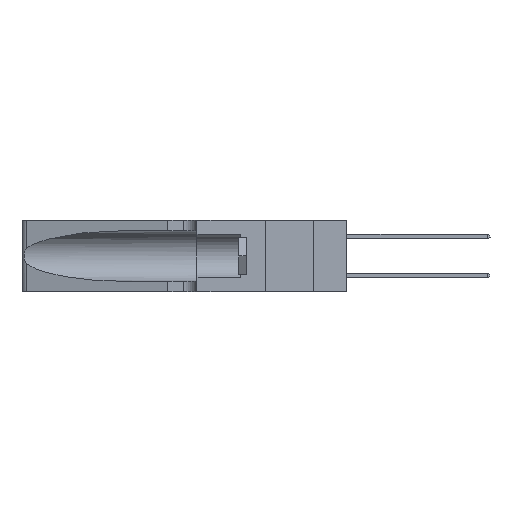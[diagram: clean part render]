
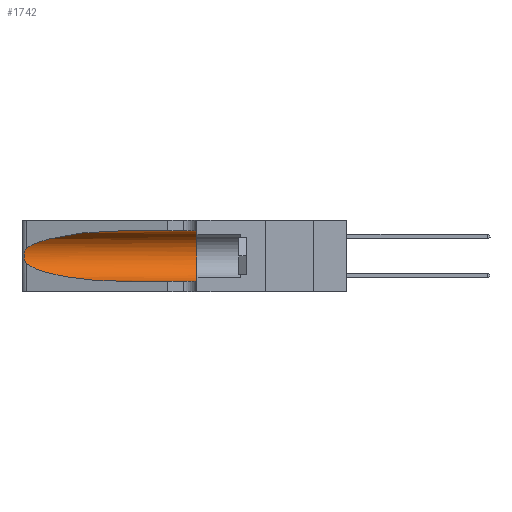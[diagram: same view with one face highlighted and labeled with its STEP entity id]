
A CAD part, left-side view. The second image highlights one B-rep face of the part: STEP entity #1742.
In plain terms, the highlighted cylindrical face has radius 3.308 mm (diameter 6.617 mm), a partial arc.
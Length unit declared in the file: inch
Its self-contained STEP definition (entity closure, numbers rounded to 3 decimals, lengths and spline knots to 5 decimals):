
#108 = CARTESIAN_POINT ( 'NONE',  ( 0.25487, 1.22718, 0.22369 ) ) ;
#180 = EDGE_CURVE ( 'NONE', #36147, #35010, #6862, .T. ) ;
#284 = DIRECTION ( 'NONE',  ( 0., -1., 0. ) ) ;
#450 = CARTESIAN_POINT ( 'NONE',  ( 0.25555, 1.22993, 0.14849 ) ) ;
#889 = B_SPLINE_CURVE_WITH_KNOTS ( 'NONE', 3,
 ( #3472, #22132, #25233, #6663, #28378, #9851, #31493, #12985, #34604, #16064, #37727, #19160, #450, #22259 ),
 .UNSPECIFIED., .F., .F.,
 ( 4, 2, 2, 2, 2, 2, 4 ),
 ( 0., 0.00027, 0.00053, 0.00107, 0.0016, 0.00187, 0.00214 ),
 .UNSPECIFIED. ) ;
#1436 = AXIS2_PLACEMENT_3D ( 'NONE', #6630, #284, #28343 ) ;
#1742 = ADVANCED_FACE ( 'NONE', ( #29060 ), #4242, .F. ) ;
#3472 = CARTESIAN_POINT ( 'NONE',  ( 0.25487, 1.22718, 0.22369 ) ) ;
#3777 = ORIENTED_EDGE ( 'NONE', *, *, #180, .F. ) ;
#4242 = CYLINDRICAL_SURFACE ( 'NONE', #1436, 0.13025 ) ;
#4255 = ORIENTED_EDGE ( 'NONE', *, *, #27857, .T. ) ;
#5279 = VERTEX_POINT ( 'NONE', #39286 ) ;
#5410 = DIRECTION ( 'NONE',  ( 0., -1., 0. ) ) ;
#6630 = CARTESIAN_POINT ( 'NONE',  ( 0.1305, 1.61858, 0.185 ) ) ;
#6663 = CARTESIAN_POINT ( 'NONE',  ( 0.25787, 1.23484, 0.2124 ) ) ;
#6862 = CIRCLE ( 'NONE', #23560, 0.13025 ) ;
#8258 =( BOUNDED_CURVE ( )  B_SPLINE_CURVE ( 3, ( #12641, #31171, #18833, #108 ),
 .UNSPECIFIED., .F., .T. ) 
 B_SPLINE_CURVE_WITH_KNOTS ( ( 4, 4 ),
 ( 1.5708, 2.84003 ),
 .UNSPECIFIED. ) 
 CURVE ( )  GEOMETRIC_REPRESENTATION_ITEM ( )  RATIONAL_B_SPLINE_CURVE ( ( 1., 0.87, 0.87, 1. ) ) 
 REPRESENTATION_ITEM ( '' )  );
#9613 = CARTESIAN_POINT ( 'NONE',  ( 0.2373, 1.15595, 0.08982 ) ) ;
#9851 = CARTESIAN_POINT ( 'NONE',  ( 0.26018, 1.23835, 0.19895 ) ) ;
#10991 = VECTOR ( 'NONE', #5410, 39.37008 ) ;
#12144 = EDGE_CURVE ( 'NONE', #21489, #35010, #36846, .T. ) ;
#12641 = CARTESIAN_POINT ( 'NONE',  ( 0.1305, 0.72297, 0.31525 ) ) ;
#12985 = CARTESIAN_POINT ( 'NONE',  ( 0.26075, 1.23896, 0.178 ) ) ;
#14938 = CARTESIAN_POINT ( 'NONE',  ( 0.25487, 1.22718, 0.14631 ) ) ;
#15076 = CARTESIAN_POINT ( 'NONE',  ( 0.1305, 0.35, 0.31525 ) ) ;
#15141 = DIRECTION ( 'NONE',  ( 0., 0., 1. ) ) ;
#15835 = CARTESIAN_POINT ( 'NONE',  ( 0.18966, 0.96281, 0.05475 ) ) ;
#16064 = CARTESIAN_POINT ( 'NONE',  ( 0.25856, 1.23593, 0.16098 ) ) ;
#18427 = ORIENTED_EDGE ( 'NONE', *, *, #35000, .T. ) ;
#18833 = CARTESIAN_POINT ( 'NONE',  ( 0.2373, 1.15595, 0.28018 ) ) ;
#19160 = CARTESIAN_POINT ( 'NONE',  ( 0.25639, 1.23186, 0.15144 ) ) ;
#20175 = LINE ( 'NONE', #27006, #10991 ) ;
#20400 = ORIENTED_EDGE ( 'NONE', *, *, #31550, .F. ) ;
#21489 = VERTEX_POINT ( 'NONE', #27837 ) ;
#22132 = CARTESIAN_POINT ( 'NONE',  ( 0.25555, 1.22994, 0.2215 ) ) ;
#22259 = CARTESIAN_POINT ( 'NONE',  ( 0.25487, 1.22718, 0.14631 ) ) ;
#22755 = VERTEX_POINT ( 'NONE', #39965 ) ;
#23560 = AXIS2_PLACEMENT_3D ( 'NONE', #37990, #38033, #15141 ) ;
#23731 = ORIENTED_EDGE ( 'NONE', *, *, #30342, .T. ) ;
#24735 = DIRECTION ( 'NONE',  ( 0., -1., 0. ) ) ;
#25129 = CARTESIAN_POINT ( 'NONE',  ( 0.1305, 0.35, 0.05475 ) ) ;
#25233 = CARTESIAN_POINT ( 'NONE',  ( 0.25639, 1.23184, 0.21858 ) ) ;
#26670 = ORIENTED_EDGE ( 'NONE', *, *, #12144, .T. ) ;
#27006 = CARTESIAN_POINT ( 'NONE',  ( 0.1305, 1.61858, 0.31525 ) ) ;
#27837 = CARTESIAN_POINT ( 'NONE',  ( 0.1305, 0.72297, 0.05475 ) ) ;
#27857 = EDGE_CURVE ( 'NONE', #5279, #22755, #8258, .T. ) ;
#28343 = DIRECTION ( 'NONE',  ( 0., 0., -1. ) ) ;
#28378 = CARTESIAN_POINT ( 'NONE',  ( 0.25854, 1.2359, 0.20912 ) ) ;
#28617 = VECTOR ( 'NONE', #24735, 39.37008 ) ;
#29060 = FACE_OUTER_BOUND ( 'NONE', #33865, .T. ) ;
#30342 = EDGE_CURVE ( 'NONE', #22755, #40206, #889, .T. ) ;
#31171 = CARTESIAN_POINT ( 'NONE',  ( 0.18966, 0.96281, 0.31525 ) ) ;
#31269 = CARTESIAN_POINT ( 'NONE',  ( 0.25487, 1.22718, 0.14631 ) ) ;
#31493 = CARTESIAN_POINT ( 'NONE',  ( 0.26075, 1.23896, 0.19203 ) ) ;
#31550 = EDGE_CURVE ( 'NONE', #5279, #36147, #20175, .T. ) ;
#33865 = EDGE_LOOP ( 'NONE', ( #4255, #23731, #18427, #26670, #3777, #20400 ) ) ;
#33963 = CARTESIAN_POINT ( 'NONE',  ( 0.1305, 1.61858, 0.05475 ) ) ;
#34054 =( BOUNDED_CURVE ( )  B_SPLINE_CURVE ( 3, ( #31269, #9613, #15835, #37495 ),
 .UNSPECIFIED., .F., .T. ) 
 B_SPLINE_CURVE_WITH_KNOTS ( ( 4, 4 ),
 ( 3.44316, 4.71239 ),
 .UNSPECIFIED. ) 
 CURVE ( )  GEOMETRIC_REPRESENTATION_ITEM ( )  RATIONAL_B_SPLINE_CURVE ( ( 1., 0.87, 0.87, 1. ) ) 
 REPRESENTATION_ITEM ( '' )  );
#34604 = CARTESIAN_POINT ( 'NONE',  ( 0.26017, 1.23833, 0.17102 ) ) ;
#35000 = EDGE_CURVE ( 'NONE', #40206, #21489, #34054, .T. ) ;
#35010 = VERTEX_POINT ( 'NONE', #25129 ) ;
#36147 = VERTEX_POINT ( 'NONE', #15076 ) ;
#36846 = LINE ( 'NONE', #33963, #28617 ) ;
#37495 = CARTESIAN_POINT ( 'NONE',  ( 0.1305, 0.72297, 0.05475 ) ) ;
#37727 = CARTESIAN_POINT ( 'NONE',  ( 0.25789, 1.23486, 0.15765 ) ) ;
#37990 = CARTESIAN_POINT ( 'NONE',  ( 0.1305, 0.35, 0.185 ) ) ;
#38033 = DIRECTION ( 'NONE',  ( 0., 1., 0. ) ) ;
#39286 = CARTESIAN_POINT ( 'NONE',  ( 0.1305, 0.72297, 0.31525 ) ) ;
#39965 = CARTESIAN_POINT ( 'NONE',  ( 0.25487, 1.22718, 0.22369 ) ) ;
#40206 = VERTEX_POINT ( 'NONE', #14938 ) ;
